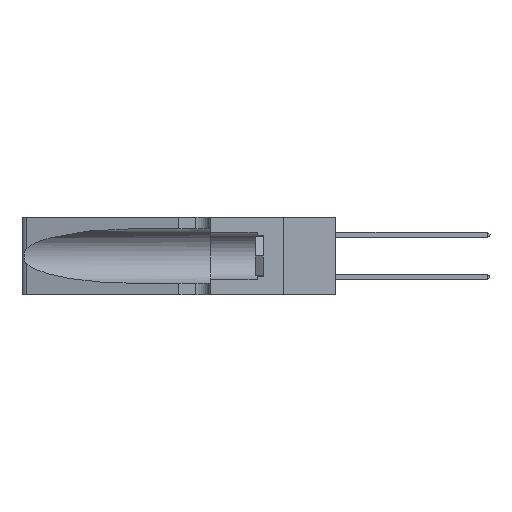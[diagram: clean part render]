
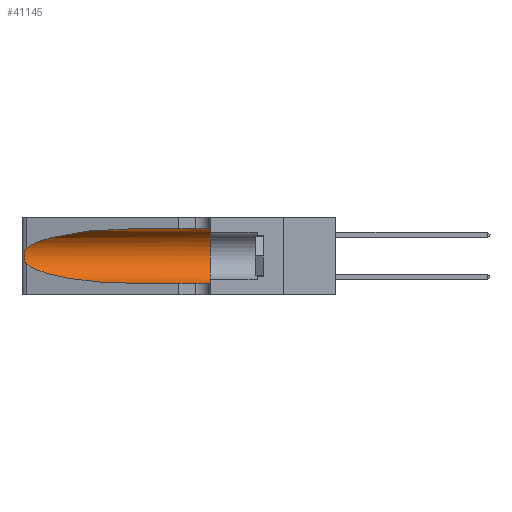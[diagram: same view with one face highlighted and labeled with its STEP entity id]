
A CAD part, left-side view. The second image highlights one B-rep face of the part: STEP entity #41145.
In plain terms, the highlighted cylindrical face has radius 3.308 mm (diameter 6.617 mm), a partial arc.
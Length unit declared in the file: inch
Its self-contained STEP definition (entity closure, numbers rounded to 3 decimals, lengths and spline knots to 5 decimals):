
#231 = CARTESIAN_POINT ( 'NONE',  ( 0.26075, 1.23896, 0.19203 ) ) ;
#1442 = ORIENTED_EDGE ( 'NONE', *, *, #25874, .T. ) ;
#2231 = VERTEX_POINT ( 'NONE', #32490 ) ;
#4784 = CARTESIAN_POINT ( 'NONE',  ( 0.25487, 1.22718, 0.22369 ) ) ;
#5741 =( BOUNDED_CURVE ( )  B_SPLINE_CURVE ( 3, ( #11902, #40557, #40833, #21669 ),
 .UNSPECIFIED., .F., .F. ) 
 B_SPLINE_CURVE_WITH_KNOTS ( ( 4, 4 ),
 ( 1.5708, 2.84003 ),
 .UNSPECIFIED. ) 
 CURVE ( )  GEOMETRIC_REPRESENTATION_ITEM ( )  RATIONAL_B_SPLINE_CURVE ( ( 1., 0.87, 0.87, 1. ) ) 
 REPRESENTATION_ITEM ( '' )  );
#5769 = EDGE_CURVE ( 'NONE', #2231, #27484, #15382, .T. ) ;
#6840 = VERTEX_POINT ( 'NONE', #4784 ) ;
#9120 = AXIS2_PLACEMENT_3D ( 'NONE', #23551, #27069, #24000 ) ;
#9729 = CARTESIAN_POINT ( 'NONE',  ( 0.25639, 1.23186, 0.15144 ) ) ;
#11902 = CARTESIAN_POINT ( 'NONE',  ( 0.1305, 0.72297, 0.31525 ) ) ;
#12338 = ORIENTED_EDGE ( 'NONE', *, *, #17334, .F. ) ;
#13040 = CARTESIAN_POINT ( 'NONE',  ( 0.25789, 1.23486, 0.15765 ) ) ;
#13114 = DIRECTION ( 'NONE',  ( 0., -1., 0. ) ) ;
#13942 = EDGE_CURVE ( 'NONE', #24393, #6840, #5741, .T. ) ;
#14145 = CARTESIAN_POINT ( 'NONE',  ( 0.1305, 0.35, 0.05475 ) ) ;
#14981 = B_SPLINE_CURVE_WITH_KNOTS ( 'NONE', 3,
 ( #35710, #29429, #38896, #32741, #16326, #29289, #231, #16733, #32606, #22690, #13040, #9729, #38634, #32220 ),
 .UNSPECIFIED., .F., .F.,
 ( 4, 2, 2, 2, 2, 2, 4 ),
 ( 0., 0.00027, 0.00053, 0.00107, 0.0016, 0.00187, 0.00214 ),
 .UNSPECIFIED. ) ;
#15027 =( BOUNDED_CURVE ( )  B_SPLINE_CURVE ( 3, ( #34334, #15083, #15625, #18876 ),
 .UNSPECIFIED., .F., .T. ) 
 B_SPLINE_CURVE_WITH_KNOTS ( ( 4, 4 ),
 ( 3.44316, 4.71239 ),
 .UNSPECIFIED. ) 
 CURVE ( )  GEOMETRIC_REPRESENTATION_ITEM ( )  RATIONAL_B_SPLINE_CURVE ( ( 1., 0.87, 0.87, 1. ) ) 
 REPRESENTATION_ITEM ( '' )  );
#15083 = CARTESIAN_POINT ( 'NONE',  ( 0.2373, 1.15595, 0.08982 ) ) ;
#15382 = CIRCLE ( 'NONE', #24817, 0.13025 ) ;
#15625 = CARTESIAN_POINT ( 'NONE',  ( 0.18966, 0.96281, 0.05475 ) ) ;
#15901 = ORIENTED_EDGE ( 'NONE', *, *, #13942, .T. ) ;
#16326 = CARTESIAN_POINT ( 'NONE',  ( 0.25854, 1.2359, 0.20912 ) ) ;
#16733 = CARTESIAN_POINT ( 'NONE',  ( 0.26075, 1.23896, 0.178 ) ) ;
#17334 = EDGE_CURVE ( 'NONE', #24393, #2231, #22924, .T. ) ;
#18568 = VECTOR ( 'NONE', #13114, 39.37008 ) ;
#18876 = CARTESIAN_POINT ( 'NONE',  ( 0.1305, 0.72297, 0.05475 ) ) ;
#19025 = DIRECTION ( 'NONE',  ( 0., -1., 0. ) ) ;
#21037 = ORIENTED_EDGE ( 'NONE', *, *, #29037, .T. ) ;
#21337 = CYLINDRICAL_SURFACE ( 'NONE', #9120, 0.13025 ) ;
#21669 = CARTESIAN_POINT ( 'NONE',  ( 0.25487, 1.22718, 0.22369 ) ) ;
#22690 = CARTESIAN_POINT ( 'NONE',  ( 0.25856, 1.23593, 0.16098 ) ) ;
#22924 = LINE ( 'NONE', #34898, #26970 ) ;
#23551 = CARTESIAN_POINT ( 'NONE',  ( 0.1305, 1.61858, 0.185 ) ) ;
#24000 = DIRECTION ( 'NONE',  ( 0., 0., -1. ) ) ;
#24001 = ORIENTED_EDGE ( 'NONE', *, *, #34332, .T. ) ;
#24393 = VERTEX_POINT ( 'NONE', #25791 ) ;
#24817 = AXIS2_PLACEMENT_3D ( 'NONE', #31087, #36822, #40454 ) ;
#25357 = FACE_OUTER_BOUND ( 'NONE', #27714, .T. ) ;
#25791 = CARTESIAN_POINT ( 'NONE',  ( 0.1305, 0.72297, 0.31525 ) ) ;
#25874 = EDGE_CURVE ( 'NONE', #37743, #27484, #27655, .T. ) ;
#26970 = VECTOR ( 'NONE', #19025, 39.37008 ) ;
#27069 = DIRECTION ( 'NONE',  ( 0., -1., 0. ) ) ;
#27484 = VERTEX_POINT ( 'NONE', #14145 ) ;
#27655 = LINE ( 'NONE', #34558, #18568 ) ;
#27714 = EDGE_LOOP ( 'NONE', ( #15901, #24001, #21037, #1442, #35881, #12338 ) ) ;
#27723 = CARTESIAN_POINT ( 'NONE',  ( 0.1305, 0.72297, 0.05475 ) ) ;
#29037 = EDGE_CURVE ( 'NONE', #38093, #37743, #15027, .T. ) ;
#29289 = CARTESIAN_POINT ( 'NONE',  ( 0.26018, 1.23835, 0.19895 ) ) ;
#29429 = CARTESIAN_POINT ( 'NONE',  ( 0.25555, 1.22994, 0.2215 ) ) ;
#31087 = CARTESIAN_POINT ( 'NONE',  ( 0.1305, 0.35, 0.185 ) ) ;
#32220 = CARTESIAN_POINT ( 'NONE',  ( 0.25487, 1.22718, 0.14631 ) ) ;
#32490 = CARTESIAN_POINT ( 'NONE',  ( 0.1305, 0.35, 0.31525 ) ) ;
#32606 = CARTESIAN_POINT ( 'NONE',  ( 0.26017, 1.23833, 0.17102 ) ) ;
#32741 = CARTESIAN_POINT ( 'NONE',  ( 0.25787, 1.23484, 0.2124 ) ) ;
#34332 = EDGE_CURVE ( 'NONE', #6840, #38093, #14981, .T. ) ;
#34334 = CARTESIAN_POINT ( 'NONE',  ( 0.25487, 1.22718, 0.14631 ) ) ;
#34558 = CARTESIAN_POINT ( 'NONE',  ( 0.1305, 1.61858, 0.05475 ) ) ;
#34898 = CARTESIAN_POINT ( 'NONE',  ( 0.1305, 1.61858, 0.31525 ) ) ;
#35710 = CARTESIAN_POINT ( 'NONE',  ( 0.25487, 1.22718, 0.22369 ) ) ;
#35881 = ORIENTED_EDGE ( 'NONE', *, *, #5769, .F. ) ;
#36822 = DIRECTION ( 'NONE',  ( 0., 1., 0. ) ) ;
#37743 = VERTEX_POINT ( 'NONE', #27723 ) ;
#38093 = VERTEX_POINT ( 'NONE', #39125 ) ;
#38634 = CARTESIAN_POINT ( 'NONE',  ( 0.25555, 1.22993, 0.14849 ) ) ;
#38896 = CARTESIAN_POINT ( 'NONE',  ( 0.25639, 1.23184, 0.21858 ) ) ;
#39125 = CARTESIAN_POINT ( 'NONE',  ( 0.25487, 1.22718, 0.14631 ) ) ;
#40454 = DIRECTION ( 'NONE',  ( 0., 0., 1. ) ) ;
#40557 = CARTESIAN_POINT ( 'NONE',  ( 0.18966, 0.96281, 0.31525 ) ) ;
#40833 = CARTESIAN_POINT ( 'NONE',  ( 0.2373, 1.15595, 0.28018 ) ) ;
#41145 = ADVANCED_FACE ( 'NONE', ( #25357 ), #21337, .F. ) ;
